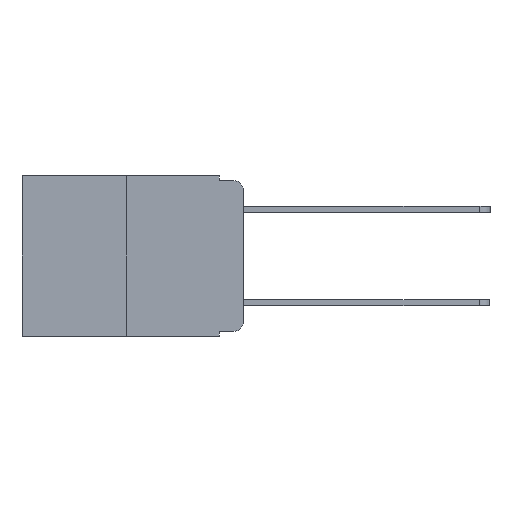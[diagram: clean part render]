
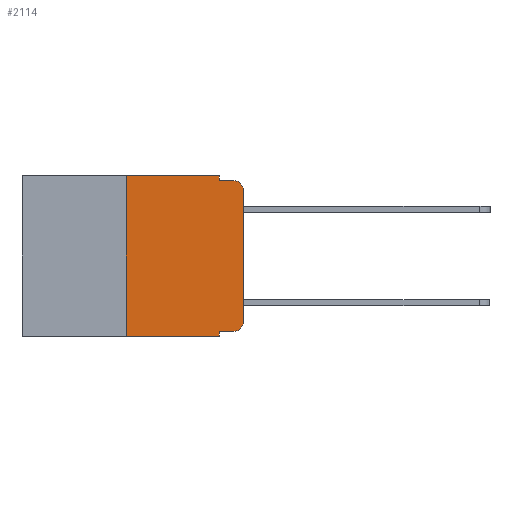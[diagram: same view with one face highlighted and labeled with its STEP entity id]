
A CAD part, left-side view. The second image highlights one B-rep face of the part: STEP entity #2114.
In plain terms, the highlighted planar face has unit normal (-1, 0, 0).
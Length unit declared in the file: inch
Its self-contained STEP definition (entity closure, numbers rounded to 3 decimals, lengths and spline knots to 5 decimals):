
#285 = DIRECTION ( 'NONE',  ( 1., 0., 0. ) ) ;
#304 = DIRECTION ( 'NONE',  ( 0., 0., 1. ) ) ;
#1416 = AXIS2_PLACEMENT_3D ( 'NONE', #9097, #285, #10602 ) ;
#1525 = DIRECTION ( 'NONE',  ( -1., 0., 0. ) ) ;
#2008 = EDGE_CURVE ( 'NONE', #14902, #13597, #2572, .T. ) ;
#2114 = ADVANCED_FACE ( 'NONE', ( #4210 ), #9038, .F. ) ;
#2489 = VECTOR ( 'NONE', #8161, 39.37008 ) ;
#2572 = CIRCLE ( 'NONE', #12639, 0.02 ) ;
#3006 = EDGE_CURVE ( 'NONE', #17304, #18509, #5568, .T. ) ;
#3122 = EDGE_CURVE ( 'NONE', #16530, #10936, #14022, .T. ) ;
#3378 = EDGE_CURVE ( 'NONE', #16408, #14902, #10808, .T. ) ;
#3600 = CARTESIAN_POINT ( 'NONE',  ( 0., 0.473, 0. ) ) ;
#4092 = ORIENTED_EDGE ( 'NONE', *, *, #11965, .F. ) ;
#4210 = FACE_OUTER_BOUND ( 'NONE', #14634, .T. ) ;
#4212 = CARTESIAN_POINT ( 'NONE',  ( 0., 0.25, -0.343 ) ) ;
#4468 = CARTESIAN_POINT ( 'NONE',  ( 0., 0.051, -0.333 ) ) ;
#4805 = VECTOR ( 'NONE', #304, 39.37008 ) ;
#5088 = EDGE_CURVE ( 'NONE', #16408, #7675, #11189, .T. ) ;
#5163 = CARTESIAN_POINT ( 'NONE',  ( 0., 0.02, -0.01 ) ) ;
#5196 = VERTEX_POINT ( 'NONE', #18779 ) ;
#5568 = LINE ( 'NONE', #15794, #11990 ) ;
#6234 = VECTOR ( 'NONE', #11747, 39.37008 ) ;
#6385 = EDGE_CURVE ( 'NONE', #5196, #11488, #15477, .T. ) ;
#6956 = DIRECTION ( 'NONE',  ( 0., 0., -1. ) ) ;
#7010 = ORIENTED_EDGE ( 'NONE', *, *, #2008, .T. ) ;
#7204 = CARTESIAN_POINT ( 'NONE',  ( 0., 0.02, -0.03 ) ) ;
#7437 = CARTESIAN_POINT ( 'NONE',  ( 0., 0.473, -0.343 ) ) ;
#7651 = CARTESIAN_POINT ( 'NONE',  ( 0., 0., 0. ) ) ;
#7675 = VERTEX_POINT ( 'NONE', #17783 ) ;
#7753 = CARTESIAN_POINT ( 'NONE',  ( 0., 0.051, 0. ) ) ;
#8161 = DIRECTION ( 'NONE',  ( 0., -1., 0. ) ) ;
#8501 = DIRECTION ( 'NONE',  ( 0., 0., -1. ) ) ;
#8677 = DIRECTION ( 'NONE',  ( 0., 0., -1. ) ) ;
#8702 = EDGE_CURVE ( 'NONE', #18509, #11488, #16797, .T. ) ;
#8753 = CARTESIAN_POINT ( 'NONE',  ( 0., 0.25, 0. ) ) ;
#9038 = PLANE ( 'NONE',  #1416 ) ;
#9097 = CARTESIAN_POINT ( 'NONE',  ( 0., 0.473, 0. ) ) ;
#9475 = VECTOR ( 'NONE', #14296, 39.37008 ) ;
#9542 = ORIENTED_EDGE ( 'NONE', *, *, #12302, .T. ) ;
#9759 = CARTESIAN_POINT ( 'NONE',  ( 0., 0.25, 0. ) ) ;
#10343 = CARTESIAN_POINT ( 'NONE',  ( 0., 0.02, -0.313 ) ) ;
#10602 = DIRECTION ( 'NONE',  ( 0., 0., -1. ) ) ;
#10808 = LINE ( 'NONE', #4468, #18035 ) ;
#10936 = VERTEX_POINT ( 'NONE', #9759 ) ;
#11060 = ORIENTED_EDGE ( 'NONE', *, *, #5088, .F. ) ;
#11189 = LINE ( 'NONE', #15715, #14631 ) ;
#11267 = ORIENTED_EDGE ( 'NONE', *, *, #3378, .T. ) ;
#11273 = ORIENTED_EDGE ( 'NONE', *, *, #8702, .F. ) ;
#11488 = VERTEX_POINT ( 'NONE', #5163 ) ;
#11747 = DIRECTION ( 'NONE',  ( 0., 0., 1. ) ) ;
#11851 = DIRECTION ( 'NONE',  ( 0., 0., -1. ) ) ;
#11965 = EDGE_CURVE ( 'NONE', #10936, #17304, #14204, .T. ) ;
#11990 = VECTOR ( 'NONE', #8501, 39.37008 ) ;
#12302 = EDGE_CURVE ( 'NONE', #13597, #5196, #16448, .T. ) ;
#12445 = AXIS2_PLACEMENT_3D ( 'NONE', #7204, #17401, #8677 ) ;
#12639 = AXIS2_PLACEMENT_3D ( 'NONE', #10343, #1525, #11851 ) ;
#12738 = LINE ( 'NONE', #7437, #16130 ) ;
#12852 = CARTESIAN_POINT ( 'NONE',  ( 0., 0.051, -0.01 ) ) ;
#12907 = ORIENTED_EDGE ( 'NONE', *, *, #14721, .T. ) ;
#13069 = ORIENTED_EDGE ( 'NONE', *, *, #3122, .F. ) ;
#13228 = CARTESIAN_POINT ( 'NONE',  ( 0., 0.051, -0.01 ) ) ;
#13548 = ORIENTED_EDGE ( 'NONE', *, *, #3006, .F. ) ;
#13597 = VERTEX_POINT ( 'NONE', #17960 ) ;
#14022 = LINE ( 'NONE', #8753, #6234 ) ;
#14204 = LINE ( 'NONE', #3600, #2489 ) ;
#14296 = DIRECTION ( 'NONE',  ( 0., -1., 0. ) ) ;
#14631 = VECTOR ( 'NONE', #6956, 39.37008 ) ;
#14634 = EDGE_LOOP ( 'NONE', ( #9542, #17686, #11273, #13548, #4092, #13069, #12907, #11060, #11267, #7010 ) ) ;
#14710 = DIRECTION ( 'NONE',  ( 0., -1., 0. ) ) ;
#14721 = EDGE_CURVE ( 'NONE', #16530, #7675, #12738, .T. ) ;
#14755 = DIRECTION ( 'NONE',  ( 0., -1., 0. ) ) ;
#14902 = VERTEX_POINT ( 'NONE', #15026 ) ;
#15026 = CARTESIAN_POINT ( 'NONE',  ( 0., 0.02, -0.333 ) ) ;
#15477 = CIRCLE ( 'NONE', #12445, 0.02 ) ;
#15647 = CARTESIAN_POINT ( 'NONE',  ( 0., 0.051, -0.333 ) ) ;
#15715 = CARTESIAN_POINT ( 'NONE',  ( 0., 0.051, 0. ) ) ;
#15794 = CARTESIAN_POINT ( 'NONE',  ( 0., 0.051, 0. ) ) ;
#16130 = VECTOR ( 'NONE', #14755, 39.37008 ) ;
#16408 = VERTEX_POINT ( 'NONE', #15647 ) ;
#16448 = LINE ( 'NONE', #7651, #4805 ) ;
#16530 = VERTEX_POINT ( 'NONE', #4212 ) ;
#16797 = LINE ( 'NONE', #12852, #9475 ) ;
#17304 = VERTEX_POINT ( 'NONE', #7753 ) ;
#17401 = DIRECTION ( 'NONE',  ( -1., 0., 0. ) ) ;
#17686 = ORIENTED_EDGE ( 'NONE', *, *, #6385, .T. ) ;
#17783 = CARTESIAN_POINT ( 'NONE',  ( 0., 0.051, -0.343 ) ) ;
#17960 = CARTESIAN_POINT ( 'NONE',  ( 0., 0., -0.313 ) ) ;
#18035 = VECTOR ( 'NONE', #14710, 39.37008 ) ;
#18509 = VERTEX_POINT ( 'NONE', #13228 ) ;
#18779 = CARTESIAN_POINT ( 'NONE',  ( 0., 0., -0.03 ) ) ;
